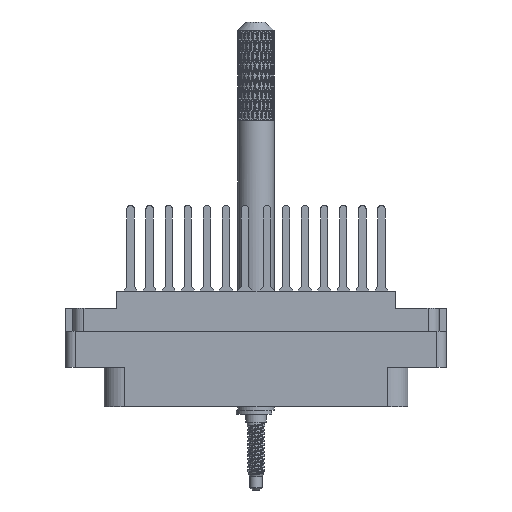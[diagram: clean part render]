
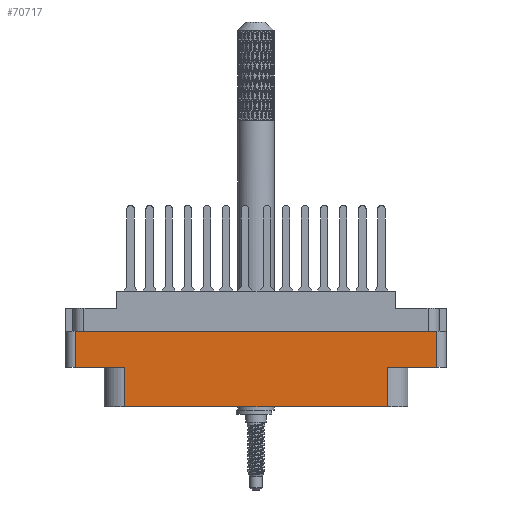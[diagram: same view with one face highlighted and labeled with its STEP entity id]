
A CAD part, front view. The second image highlights one B-rep face of the part: STEP entity #70717.
In plain terms, the highlighted planar face has unit normal (0, -1, 0).
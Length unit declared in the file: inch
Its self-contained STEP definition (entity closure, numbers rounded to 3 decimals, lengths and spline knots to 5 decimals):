
#2561 = CARTESIAN_POINT ( 'NONE',  ( -1.2335, -0.438, -0.274 ) ) ;
#3727 = DIRECTION ( 'NONE',  ( 1., 0., 0. ) ) ;
#4130 = LINE ( 'NONE', #10463, #81948 ) ;
#7655 = VECTOR ( 'NONE', #93283, 39.37008 ) ;
#7702 = DIRECTION ( 'NONE',  ( 0., 0., -1. ) ) ;
#10463 = CARTESIAN_POINT ( 'NONE',  ( 0., -0.438, -0.52 ) ) ;
#12182 = CARTESIAN_POINT ( 'NONE',  ( -1.2335, -0.438, -0.52 ) ) ;
#12395 = CARTESIAN_POINT ( 'NONE',  ( 0.895, -0.438, -0.52 ) ) ;
#12406 = ORIENTED_EDGE ( 'NONE', *, *, #38812, .T. ) ;
#12602 = EDGE_LOOP ( 'NONE', ( #69652, #12406, #30164, #71570, #100689, #112376, #35152, #47668 ) ) ;
#12826 = VECTOR ( 'NONE', #37130, 39.37008 ) ;
#13867 = LINE ( 'NONE', #74929, #88857 ) ;
#13869 = VERTEX_POINT ( 'NONE', #2561 ) ;
#17667 = EDGE_CURVE ( 'NONE', #107753, #108598, #55538, .T. ) ;
#17762 = VERTEX_POINT ( 'NONE', #41804 ) ;
#18084 = LINE ( 'NONE', #83735, #72104 ) ;
#18653 = EDGE_CURVE ( 'NONE', #13869, #79282, #18084, .T. ) ;
#23017 = CARTESIAN_POINT ( 'NONE',  ( 1.2335, -0.438, -0.789 ) ) ;
#27414 = VERTEX_POINT ( 'NONE', #12182 ) ;
#30164 = ORIENTED_EDGE ( 'NONE', *, *, #34398, .F. ) ;
#34398 = EDGE_CURVE ( 'NONE', #17762, #27414, #107290, .T. ) ;
#34699 = CARTESIAN_POINT ( 'NONE',  ( 0.895, -0.438, -0.52 ) ) ;
#35152 = ORIENTED_EDGE ( 'NONE', *, *, #49287, .F. ) ;
#37130 = DIRECTION ( 'NONE',  ( -1., 0., 0. ) ) ;
#38812 = EDGE_CURVE ( 'NONE', #13869, #27414, #91490, .T. ) ;
#40340 = VERTEX_POINT ( 'NONE', #96778 ) ;
#41682 = EDGE_CURVE ( 'NONE', #40340, #79282, #57611, .T. ) ;
#41804 = CARTESIAN_POINT ( 'NONE',  ( -0.895, -0.438, -0.52 ) ) ;
#47668 = ORIENTED_EDGE ( 'NONE', *, *, #41682, .T. ) ;
#47826 = EDGE_CURVE ( 'NONE', #108598, #56311, #62748, .T. ) ;
#49287 = EDGE_CURVE ( 'NONE', #40340, #56311, #4130, .T. ) ;
#55538 = LINE ( 'NONE', #91968, #58357 ) ;
#56311 = VERTEX_POINT ( 'NONE', #34699 ) ;
#57611 = LINE ( 'NONE', #23017, #7655 ) ;
#58357 = VECTOR ( 'NONE', #3727, 39.37008 ) ;
#60837 = DIRECTION ( 'NONE',  ( 0., -1., 0. ) ) ;
#62748 = LINE ( 'NONE', #12395, #82290 ) ;
#62965 = CARTESIAN_POINT ( 'NONE',  ( 0.895, -0.438, -0.789 ) ) ;
#63444 = CARTESIAN_POINT ( 'NONE',  ( 0., -0.438, -0.52 ) ) ;
#64311 = DIRECTION ( 'NONE',  ( -1., 0., 0. ) ) ;
#66638 = DIRECTION ( 'NONE',  ( 0., 0., 1. ) ) ;
#66781 = CARTESIAN_POINT ( 'NONE',  ( -1.2335, -0.438, -0.789 ) ) ;
#67162 = DIRECTION ( 'NONE',  ( 0., 0., -1. ) ) ;
#69652 = ORIENTED_EDGE ( 'NONE', *, *, #18653, .F. ) ;
#70717 = ADVANCED_FACE ( 'NONE', ( #79283 ), #105227, .T. ) ;
#71570 = ORIENTED_EDGE ( 'NONE', *, *, #73439, .T. ) ;
#72104 = VECTOR ( 'NONE', #75529, 39.37008 ) ;
#73439 = EDGE_CURVE ( 'NONE', #17762, #107753, #13867, .T. ) ;
#74929 = CARTESIAN_POINT ( 'NONE',  ( -0.895, -0.438, -0.789 ) ) ;
#75529 = DIRECTION ( 'NONE',  ( 1., 0., 0. ) ) ;
#79282 = VERTEX_POINT ( 'NONE', #81792 ) ;
#79283 = FACE_OUTER_BOUND ( 'NONE', #12602, .T. ) ;
#81792 = CARTESIAN_POINT ( 'NONE',  ( 1.2335, -0.438, -0.274 ) ) ;
#81948 = VECTOR ( 'NONE', #64311, 39.37008 ) ;
#82290 = VECTOR ( 'NONE', #66638, 39.37008 ) ;
#83735 = CARTESIAN_POINT ( 'NONE',  ( 0., -0.438, -0.274 ) ) ;
#84180 = AXIS2_PLACEMENT_3D ( 'NONE', #96273, #60837, #7702 ) ;
#88857 = VECTOR ( 'NONE', #111914, 39.37008 ) ;
#90170 = VECTOR ( 'NONE', #67162, 39.37008 ) ;
#91490 = LINE ( 'NONE', #66781, #90170 ) ;
#91968 = CARTESIAN_POINT ( 'NONE',  ( -1.2955, -0.438, -0.789 ) ) ;
#93283 = DIRECTION ( 'NONE',  ( 0., 0., 1. ) ) ;
#96273 = CARTESIAN_POINT ( 'NONE',  ( -1.2955, -0.438, -0.789 ) ) ;
#96778 = CARTESIAN_POINT ( 'NONE',  ( 1.2335, -0.438, -0.52 ) ) ;
#100689 = ORIENTED_EDGE ( 'NONE', *, *, #17667, .T. ) ;
#102782 = CARTESIAN_POINT ( 'NONE',  ( -0.895, -0.438, -0.789 ) ) ;
#105227 = PLANE ( 'NONE',  #84180 ) ;
#107290 = LINE ( 'NONE', #63444, #12826 ) ;
#107753 = VERTEX_POINT ( 'NONE', #102782 ) ;
#108598 = VERTEX_POINT ( 'NONE', #62965 ) ;
#111914 = DIRECTION ( 'NONE',  ( 0., 0., -1. ) ) ;
#112376 = ORIENTED_EDGE ( 'NONE', *, *, #47826, .T. ) ;
